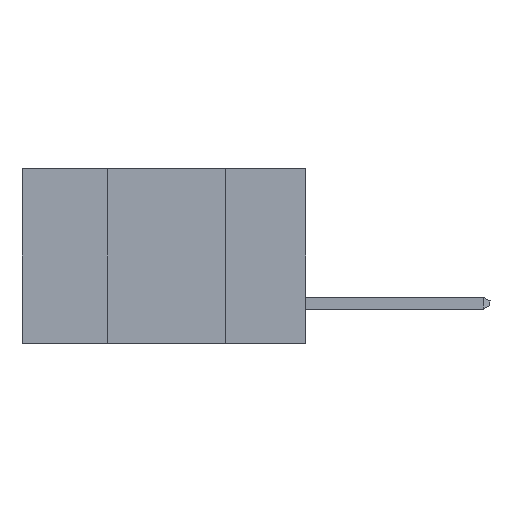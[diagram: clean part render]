
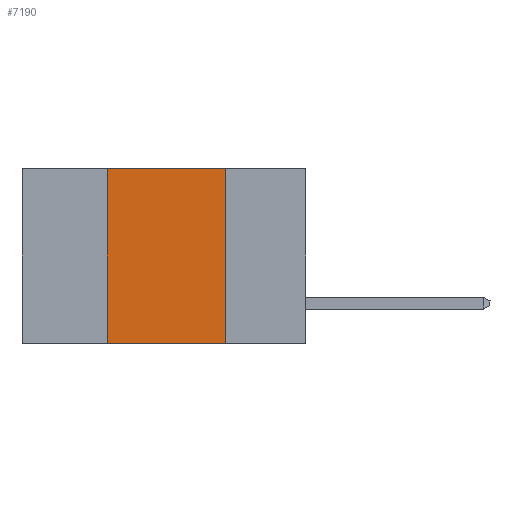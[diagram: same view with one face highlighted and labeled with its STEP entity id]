
A CAD part, left-side view. The second image highlights one B-rep face of the part: STEP entity #7190.
In plain terms, the highlighted planar face has unit normal (-1, 0, 0).
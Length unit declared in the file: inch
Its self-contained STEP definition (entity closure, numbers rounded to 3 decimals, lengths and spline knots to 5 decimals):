
#264 = VERTEX_POINT ( 'NONE', #4652 ) ;
#383 = LINE ( 'NONE', #6745, #5446 ) ;
#727 = DIRECTION ( 'NONE',  ( 0., 0., -1. ) ) ;
#820 = CARTESIAN_POINT ( 'NONE',  ( 0., 0.6, -0.37 ) ) ;
#1332 = CARTESIAN_POINT ( 'NONE',  ( 0., 0.6, 0. ) ) ;
#1690 = DIRECTION ( 'NONE',  ( 1., 0., 0. ) ) ;
#1715 = ORIENTED_EDGE ( 'NONE', *, *, #12325, .F. ) ;
#2392 = CARTESIAN_POINT ( 'NONE',  ( 0., 0.17, -0.37 ) ) ;
#2399 = ORIENTED_EDGE ( 'NONE', *, *, #2699, .F. ) ;
#2699 = EDGE_CURVE ( 'NONE', #12341, #3834, #12862, .T. ) ;
#3834 = VERTEX_POINT ( 'NONE', #2392 ) ;
#4156 = EDGE_CURVE ( 'NONE', #12886, #12341, #6454, .T. ) ;
#4505 = DIRECTION ( 'NONE',  ( 0., -1., 0. ) ) ;
#4652 = CARTESIAN_POINT ( 'NONE',  ( 0., 0.42, -0.37 ) ) ;
#5030 = CARTESIAN_POINT ( 'NONE',  ( 0., 0.17, -0.37 ) ) ;
#5446 = VECTOR ( 'NONE', #5676, 39.37008 ) ;
#5676 = DIRECTION ( 'NONE',  ( 0., 0., 1. ) ) ;
#5684 = PLANE ( 'NONE',  #12018 ) ;
#5692 = VECTOR ( 'NONE', #4505, 39.37008 ) ;
#5894 = CARTESIAN_POINT ( 'NONE',  ( 0., 0.17, 0. ) ) ;
#5899 = VECTOR ( 'NONE', #6060, 39.37008 ) ;
#6060 = DIRECTION ( 'NONE',  ( 0., -1., 0. ) ) ;
#6454 = LINE ( 'NONE', #1332, #5692 ) ;
#6745 = CARTESIAN_POINT ( 'NONE',  ( 0., 0.42, -0.37 ) ) ;
#7190 = ADVANCED_FACE ( 'NONE', ( #11425 ), #5684, .F. ) ;
#7440 = EDGE_LOOP ( 'NONE', ( #2399, #9597, #1715, #7674 ) ) ;
#7674 = ORIENTED_EDGE ( 'NONE', *, *, #13349, .T. ) ;
#9287 = DIRECTION ( 'NONE',  ( 0., 0., -1. ) ) ;
#9597 = ORIENTED_EDGE ( 'NONE', *, *, #4156, .F. ) ;
#9928 = VECTOR ( 'NONE', #727, 39.37008 ) ;
#10610 = CARTESIAN_POINT ( 'NONE',  ( 0., 0.42, 0. ) ) ;
#11425 = FACE_OUTER_BOUND ( 'NONE', #7440, .T. ) ;
#11454 = LINE ( 'NONE', #820, #5899 ) ;
#12018 = AXIS2_PLACEMENT_3D ( 'NONE', #12226, #1690, #9287 ) ;
#12226 = CARTESIAN_POINT ( 'NONE',  ( 0., 0.6, 0. ) ) ;
#12325 = EDGE_CURVE ( 'NONE', #264, #12886, #383, .T. ) ;
#12341 = VERTEX_POINT ( 'NONE', #5894 ) ;
#12862 = LINE ( 'NONE', #5030, #9928 ) ;
#12886 = VERTEX_POINT ( 'NONE', #10610 ) ;
#13349 = EDGE_CURVE ( 'NONE', #264, #3834, #11454, .T. ) ;
